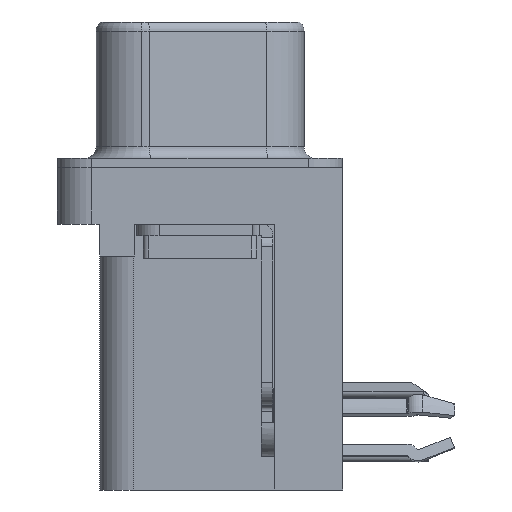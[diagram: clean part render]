
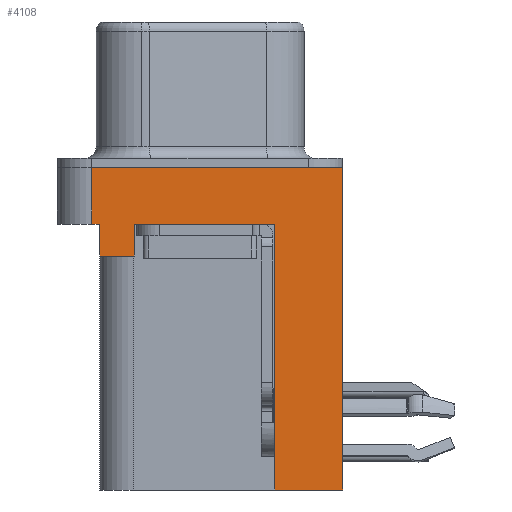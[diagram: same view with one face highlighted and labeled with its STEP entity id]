
A CAD part, left-side view. The second image highlights one B-rep face of the part: STEP entity #4108.
In plain terms, the highlighted planar face has unit normal (-1, 0, 0).
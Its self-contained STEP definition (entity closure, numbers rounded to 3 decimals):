
#33 = ORIENTED_EDGE ( 'NONE', *, *, #18719, .T. ) ;
#333 = VECTOR ( 'NONE', #13941, 1000. ) ;
#579 = CARTESIAN_POINT ( 'NONE',  ( -2.935, 4.775, -2.5 ) ) ;
#586 = LINE ( 'NONE', #19641, #9793 ) ;
#806 = LINE ( 'NONE', #8443, #15410 ) ;
#989 = ORIENTED_EDGE ( 'NONE', *, *, #17679, .F. ) ;
#1130 = VERTEX_POINT ( 'NONE', #13735 ) ;
#1153 = LINE ( 'NONE', #12503, #17163 ) ;
#1239 = ORIENTED_EDGE ( 'NONE', *, *, #14263, .F. ) ;
#1274 = EDGE_CURVE ( 'NONE', #2980, #2224, #12392, .T. ) ;
#1770 = CARTESIAN_POINT ( 'NONE',  ( -2.935, 2.895, -2.5 ) ) ;
#1791 = ORIENTED_EDGE ( 'NONE', *, *, #10865, .F. ) ;
#2012 = LINE ( 'NONE', #16254, #7311 ) ;
#2084 = DIRECTION ( 'NONE',  ( 0., 0., 1. ) ) ;
#2154 = ORIENTED_EDGE ( 'NONE', *, *, #18284, .T. ) ;
#2224 = VERTEX_POINT ( 'NONE', #14576 ) ;
#2251 = DIRECTION ( 'NONE',  ( 0., 0., 1. ) ) ;
#2378 = EDGE_CURVE ( 'NONE', #7419, #10260, #18261, .T. ) ;
#2456 = EDGE_CURVE ( 'NONE', #1130, #9350, #1153, .T. ) ;
#2568 = DIRECTION ( 'NONE',  ( -1., 0., 0. ) ) ;
#2980 = VERTEX_POINT ( 'NONE', #15156 ) ;
#3013 = DIRECTION ( 'NONE',  ( 0., -1., 0. ) ) ;
#3120 = AXIS2_PLACEMENT_3D ( 'NONE', #16492, #2568, #13317 ) ;
#4010 = PLANE ( 'NONE',  #3120 ) ;
#4108 = ADVANCED_FACE ( 'NONE', ( #6819 ), #4010, .T. ) ;
#4315 = CARTESIAN_POINT ( 'NONE',  ( -2.935, 4.425, -2.5 ) ) ;
#4851 = LINE ( 'NONE', #8043, #19225 ) ;
#5133 = VECTOR ( 'NONE', #13799, 1000. ) ;
#5332 = DIRECTION ( 'NONE',  ( 0., -1., 0. ) ) ;
#6038 = ORIENTED_EDGE ( 'NONE', *, *, #1274, .F. ) ;
#6556 = ORIENTED_EDGE ( 'NONE', *, *, #9758, .F. ) ;
#6819 = FACE_OUTER_BOUND ( 'NONE', #14182, .T. ) ;
#6916 = DIRECTION ( 'NONE',  ( 0., 0., 1. ) ) ;
#6941 = CARTESIAN_POINT ( 'NONE',  ( -2.935, 2.895, -3.9 ) ) ;
#7311 = VECTOR ( 'NONE', #14610, 1000. ) ;
#7419 = VERTEX_POINT ( 'NONE', #17648 ) ;
#7643 = CARTESIAN_POINT ( 'NONE',  ( -2.935, -6.275, 0. ) ) ;
#8043 = CARTESIAN_POINT ( 'NONE',  ( -2.935, -3.295, -14.2 ) ) ;
#8443 = CARTESIAN_POINT ( 'NONE',  ( -2.935, -6.275, -2.5 ) ) ;
#9350 = VERTEX_POINT ( 'NONE', #4315 ) ;
#9627 = LINE ( 'NONE', #14087, #14068 ) ;
#9758 = EDGE_CURVE ( 'NONE', #7419, #1130, #20263, .T. ) ;
#9793 = VECTOR ( 'NONE', #5332, 1000. ) ;
#9968 = VERTEX_POINT ( 'NONE', #17275 ) ;
#10260 = VERTEX_POINT ( 'NONE', #1770 ) ;
#10366 = CARTESIAN_POINT ( 'NONE',  ( -2.935, -6.275, -14.2 ) ) ;
#10532 = DIRECTION ( 'NONE',  ( 0., 0., 1. ) ) ;
#10562 = ORIENTED_EDGE ( 'NONE', *, *, #19627, .T. ) ;
#10805 = VERTEX_POINT ( 'NONE', #579 ) ;
#10855 = LINE ( 'NONE', #17135, #19336 ) ;
#10865 = EDGE_CURVE ( 'NONE', #16047, #12333, #2012, .T. ) ;
#10912 = ORIENTED_EDGE ( 'NONE', *, *, #2378, .T. ) ;
#12333 = VERTEX_POINT ( 'NONE', #18707 ) ;
#12392 = LINE ( 'NONE', #7643, #333 ) ;
#12503 = CARTESIAN_POINT ( 'NONE',  ( -2.935, 4.425, -3.9 ) ) ;
#12538 = DIRECTION ( 'NONE',  ( 0., 0., 1. ) ) ;
#12897 = VECTOR ( 'NONE', #2084, 1000. ) ;
#13317 = DIRECTION ( 'NONE',  ( 0., 0., 1. ) ) ;
#13735 = CARTESIAN_POINT ( 'NONE',  ( -2.935, 4.425, -3.9 ) ) ;
#13799 = DIRECTION ( 'NONE',  ( 0., 1., 0. ) ) ;
#13941 = DIRECTION ( 'NONE',  ( 0., -1., 0. ) ) ;
#14068 = VECTOR ( 'NONE', #12538, 1000. ) ;
#14087 = CARTESIAN_POINT ( 'NONE',  ( -2.935, 4.775, -2.5 ) ) ;
#14182 = EDGE_LOOP ( 'NONE', ( #6038, #989, #10562, #18039, #6556, #10912, #33, #1239, #1791, #2154 ) ) ;
#14263 = EDGE_CURVE ( 'NONE', #12333, #9968, #4851, .T. ) ;
#14576 = CARTESIAN_POINT ( 'NONE',  ( -2.935, -6.275, 0. ) ) ;
#14610 = DIRECTION ( 'NONE',  ( 0., 1., 0. ) ) ;
#15156 = CARTESIAN_POINT ( 'NONE',  ( -2.935, 4.775, 0. ) ) ;
#15410 = VECTOR ( 'NONE', #2251, 1000. ) ;
#15436 = CARTESIAN_POINT ( 'NONE',  ( -2.935, 4.425, -3.9 ) ) ;
#16047 = VERTEX_POINT ( 'NONE', #10366 ) ;
#16254 = CARTESIAN_POINT ( 'NONE',  ( -2.935, -3.295, -14.2 ) ) ;
#16492 = CARTESIAN_POINT ( 'NONE',  ( -2.935, -6.275, -2.5 ) ) ;
#17135 = CARTESIAN_POINT ( 'NONE',  ( -2.935, -6.275, -2.5 ) ) ;
#17163 = VECTOR ( 'NONE', #10532, 1000. ) ;
#17275 = CARTESIAN_POINT ( 'NONE',  ( -2.935, -3.295, -2.5 ) ) ;
#17648 = CARTESIAN_POINT ( 'NONE',  ( -2.935, 2.895, -3.9 ) ) ;
#17679 = EDGE_CURVE ( 'NONE', #10805, #2980, #9627, .T. ) ;
#18039 = ORIENTED_EDGE ( 'NONE', *, *, #2456, .F. ) ;
#18261 = LINE ( 'NONE', #6941, #12897 ) ;
#18284 = EDGE_CURVE ( 'NONE', #16047, #2224, #806, .T. ) ;
#18707 = CARTESIAN_POINT ( 'NONE',  ( -2.935, -3.295, -14.2 ) ) ;
#18719 = EDGE_CURVE ( 'NONE', #10260, #9968, #586, .T. ) ;
#19225 = VECTOR ( 'NONE', #6916, 1000. ) ;
#19336 = VECTOR ( 'NONE', #3013, 1000. ) ;
#19627 = EDGE_CURVE ( 'NONE', #10805, #9350, #10855, .T. ) ;
#19641 = CARTESIAN_POINT ( 'NONE',  ( -2.935, -6.275, -2.5 ) ) ;
#20263 = LINE ( 'NONE', #15436, #5133 ) ;
